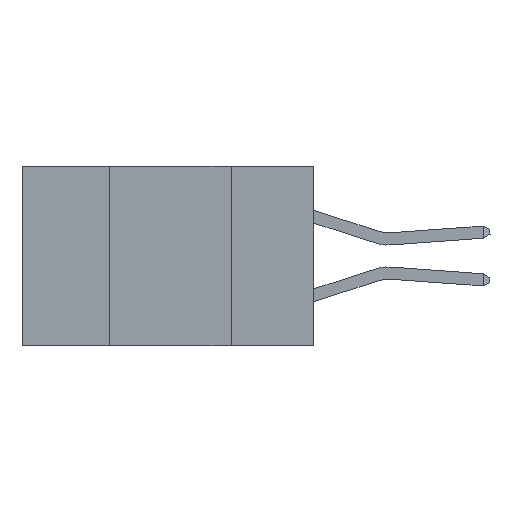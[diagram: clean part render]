
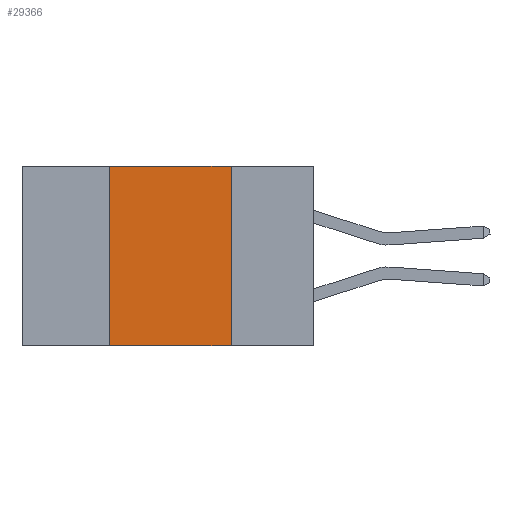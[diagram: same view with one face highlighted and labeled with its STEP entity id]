
A CAD part, left-side view. The second image highlights one B-rep face of the part: STEP entity #29366.
In plain terms, the highlighted planar face has unit normal (-1, 0, 0).
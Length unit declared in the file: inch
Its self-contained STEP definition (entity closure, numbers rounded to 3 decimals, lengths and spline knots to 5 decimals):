
#117 = ORIENTED_EDGE ( 'NONE', *, *, #32083, .F. ) ;
#790 = CARTESIAN_POINT ( 'NONE',  ( 0., 0.6, 0. ) ) ;
#2564 = ORIENTED_EDGE ( 'NONE', *, *, #34937, .F. ) ;
#2751 = DIRECTION ( 'NONE',  ( 0., 0., 1. ) ) ;
#2910 = EDGE_CURVE ( 'NONE', #31707, #16480, #24685, .T. ) ;
#3729 = LINE ( 'NONE', #790, #7687 ) ;
#5027 = CARTESIAN_POINT ( 'NONE',  ( 0., 0.17, -0.37 ) ) ;
#5142 = EDGE_CURVE ( 'NONE', #6533, #16480, #6058, .T. ) ;
#5247 = CARTESIAN_POINT ( 'NONE',  ( 0., 0.6, -0.37 ) ) ;
#5892 = PLANE ( 'NONE',  #31511 ) ;
#5900 = CARTESIAN_POINT ( 'NONE',  ( 0., 0.42, -0.37 ) ) ;
#6058 = LINE ( 'NONE', #14147, #8302 ) ;
#6533 = VERTEX_POINT ( 'NONE', #19161 ) ;
#6803 = ORIENTED_EDGE ( 'NONE', *, *, #2910, .T. ) ;
#7687 = VECTOR ( 'NONE', #28305, 39.37008 ) ;
#8302 = VECTOR ( 'NONE', #34489, 39.37008 ) ;
#8405 = VECTOR ( 'NONE', #19580, 39.37008 ) ;
#9543 = DIRECTION ( 'NONE',  ( 0., 0., -1. ) ) ;
#11428 = ORIENTED_EDGE ( 'NONE', *, *, #5142, .F. ) ;
#12110 = EDGE_LOOP ( 'NONE', ( #11428, #2564, #117, #6803 ) ) ;
#14147 = CARTESIAN_POINT ( 'NONE',  ( 0., 0.17, 0. ) ) ;
#15059 = VERTEX_POINT ( 'NONE', #23917 ) ;
#16480 = VERTEX_POINT ( 'NONE', #5027 ) ;
#16885 = CARTESIAN_POINT ( 'NONE',  ( 0., 0.42, 0. ) ) ;
#19161 = CARTESIAN_POINT ( 'NONE',  ( 0., 0.17, 0. ) ) ;
#19580 = DIRECTION ( 'NONE',  ( 0., -1., 0. ) ) ;
#21574 = VECTOR ( 'NONE', #2751, 39.37008 ) ;
#23917 = CARTESIAN_POINT ( 'NONE',  ( 0., 0.42, 0. ) ) ;
#24010 = CARTESIAN_POINT ( 'NONE',  ( 0., 0.6, 0. ) ) ;
#24685 = LINE ( 'NONE', #5247, #8405 ) ;
#26760 = DIRECTION ( 'NONE',  ( 1., 0., 0. ) ) ;
#28240 = LINE ( 'NONE', #16885, #21574 ) ;
#28305 = DIRECTION ( 'NONE',  ( 0., -1., 0. ) ) ;
#29366 = ADVANCED_FACE ( 'NONE', ( #34496 ), #5892, .F. ) ;
#31511 = AXIS2_PLACEMENT_3D ( 'NONE', #24010, #26760, #9543 ) ;
#31707 = VERTEX_POINT ( 'NONE', #5900 ) ;
#32083 = EDGE_CURVE ( 'NONE', #31707, #15059, #28240, .T. ) ;
#34489 = DIRECTION ( 'NONE',  ( 0., 0., -1. ) ) ;
#34496 = FACE_OUTER_BOUND ( 'NONE', #12110, .T. ) ;
#34937 = EDGE_CURVE ( 'NONE', #15059, #6533, #3729, .T. ) ;
